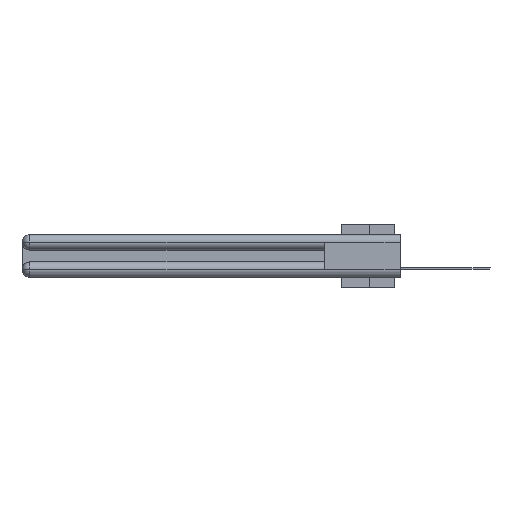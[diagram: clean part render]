
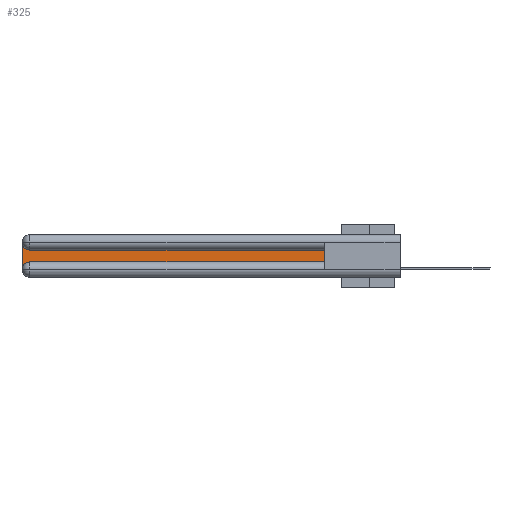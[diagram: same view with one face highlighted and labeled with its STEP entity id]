
A CAD part, left-side view. The second image highlights one B-rep face of the part: STEP entity #325.
In plain terms, the highlighted planar face has unit normal (-1, 0, 0).
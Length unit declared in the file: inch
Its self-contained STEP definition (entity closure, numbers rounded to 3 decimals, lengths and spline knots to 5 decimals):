
#58 = EDGE_CURVE ( 'NONE', #20537, #33563, #27408, .T. ) ;
#325 = ADVANCED_FACE ( 'NONE', ( #8532 ), #32684, .F. ) ;
#3403 = DIRECTION ( 'NONE',  ( 1., 0., 0. ) ) ;
#3519 = DIRECTION ( 'NONE',  ( 0., 0., 1. ) ) ;
#3965 = EDGE_CURVE ( 'NONE', #19213, #34958, #18901, .T. ) ;
#5302 = CARTESIAN_POINT ( 'NONE',  ( 0.075, 0.6, -0.2175 ) ) ;
#5597 = VERTEX_POINT ( 'NONE', #21294 ) ;
#6416 = EDGE_LOOP ( 'NONE', ( #27514, #14269, #9210, #17737, #33571, #19872 ) ) ;
#7703 = EDGE_CURVE ( 'NONE', #17630, #5597, #30935, .T. ) ;
#7767 = LINE ( 'NONE', #30389, #30027 ) ;
#8105 = DIRECTION ( 'NONE',  ( 1., 0., 0. ) ) ;
#8532 = FACE_OUTER_BOUND ( 'NONE', #6416, .T. ) ;
#9210 = ORIENTED_EDGE ( 'NONE', *, *, #9684, .T. ) ;
#9684 = EDGE_CURVE ( 'NONE', #5597, #19213, #7767, .T. ) ;
#13387 = DIRECTION ( 'NONE',  ( 0., 0., -1. ) ) ;
#13548 = DIRECTION ( 'NONE',  ( 0., 0., -1. ) ) ;
#13899 = CARTESIAN_POINT ( 'NONE',  ( 0.075, 0.6, -0.1225 ) ) ;
#14269 = ORIENTED_EDGE ( 'NONE', *, *, #7703, .T. ) ;
#14285 = AXIS2_PLACEMENT_3D ( 'NONE', #24905, #8105, #13387 ) ;
#16385 = CARTESIAN_POINT ( 'NONE',  ( 0.075, 2.94, -0.1225 ) ) ;
#16428 = EDGE_CURVE ( 'NONE', #34958, #20537, #35044, .T. ) ;
#16872 = VECTOR ( 'NONE', #3519, 39.37008 ) ;
#17297 = CARTESIAN_POINT ( 'NONE',  ( 0.075, 2.94, -0.0625 ) ) ;
#17630 = VERTEX_POINT ( 'NONE', #16385 ) ;
#17737 = ORIENTED_EDGE ( 'NONE', *, *, #3965, .T. ) ;
#18901 = CIRCLE ( 'NONE', #20455, 0.06 ) ;
#19022 = DIRECTION ( 'NONE',  ( 0., 0., -1. ) ) ;
#19213 = VERTEX_POINT ( 'NONE', #29488 ) ;
#19872 = ORIENTED_EDGE ( 'NONE', *, *, #58, .T. ) ;
#19998 = DIRECTION ( 'NONE',  ( 0., -1., 0. ) ) ;
#20455 = AXIS2_PLACEMENT_3D ( 'NONE', #20838, #23675, #19022 ) ;
#20537 = VERTEX_POINT ( 'NONE', #21879 ) ;
#20838 = CARTESIAN_POINT ( 'NONE',  ( 0.075, 2.94, -0.2775 ) ) ;
#21090 = DIRECTION ( 'NONE',  ( 0., 0., -1. ) ) ;
#21294 = CARTESIAN_POINT ( 'NONE',  ( 0.075, 3., -0.0625 ) ) ;
#21879 = CARTESIAN_POINT ( 'NONE',  ( 0.075, 0.6, -0.2175 ) ) ;
#22454 = AXIS2_PLACEMENT_3D ( 'NONE', #17297, #3403, #21090 ) ;
#23461 = LINE ( 'NONE', #27240, #34522 ) ;
#23675 = DIRECTION ( 'NONE',  ( 1., 0., 0. ) ) ;
#24905 = CARTESIAN_POINT ( 'NONE',  ( 0.075, 3., -0.1225 ) ) ;
#25642 = CARTESIAN_POINT ( 'NONE',  ( 0.075, 0.6, -0.2175 ) ) ;
#27240 = CARTESIAN_POINT ( 'NONE',  ( 0.075, 0.6, -0.1225 ) ) ;
#27408 = LINE ( 'NONE', #25642, #16872 ) ;
#27514 = ORIENTED_EDGE ( 'NONE', *, *, #32182, .T. ) ;
#29488 = CARTESIAN_POINT ( 'NONE',  ( 0.075, 3., -0.2775 ) ) ;
#30027 = VECTOR ( 'NONE', #13548, 39.37008 ) ;
#30389 = CARTESIAN_POINT ( 'NONE',  ( 0.075, 3., -0.2175 ) ) ;
#30935 = CIRCLE ( 'NONE', #22454, 0.06 ) ;
#32182 = EDGE_CURVE ( 'NONE', #33563, #17630, #23461, .T. ) ;
#32681 = DIRECTION ( 'NONE',  ( 0., 1., 0. ) ) ;
#32684 = PLANE ( 'NONE',  #14285 ) ;
#33563 = VERTEX_POINT ( 'NONE', #13899 ) ;
#33571 = ORIENTED_EDGE ( 'NONE', *, *, #16428, .T. ) ;
#33903 = CARTESIAN_POINT ( 'NONE',  ( 0.075, 2.94, -0.2175 ) ) ;
#34522 = VECTOR ( 'NONE', #32681, 39.37008 ) ;
#34958 = VERTEX_POINT ( 'NONE', #33903 ) ;
#35044 = LINE ( 'NONE', #5302, #35525 ) ;
#35525 = VECTOR ( 'NONE', #19998, 39.37008 ) ;
